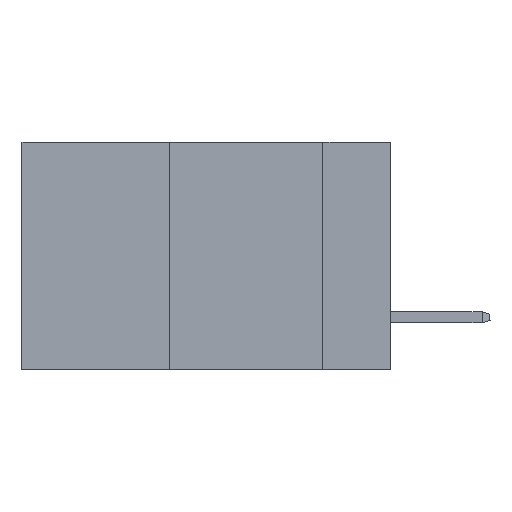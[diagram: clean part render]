
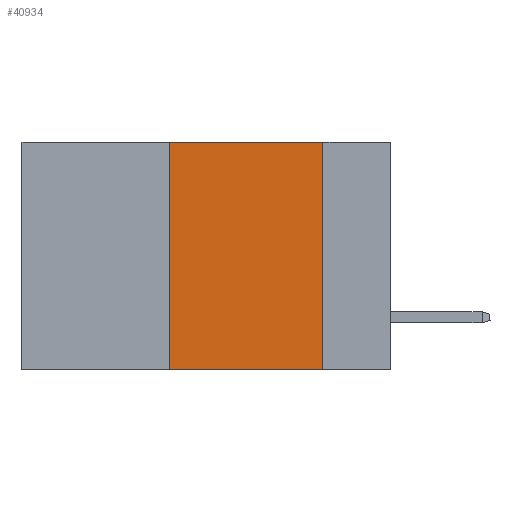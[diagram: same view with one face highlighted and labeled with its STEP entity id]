
A CAD part, left-side view. The second image highlights one B-rep face of the part: STEP entity #40934.
In plain terms, the highlighted planar face has unit normal (-1, 0, 0).
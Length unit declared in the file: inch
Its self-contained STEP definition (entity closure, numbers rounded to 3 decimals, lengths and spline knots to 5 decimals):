
#1738 = DIRECTION ( 'NONE',  ( 0., 0., 1. ) ) ;
#4378 = EDGE_CURVE ( 'NONE', #25977, #31112, #27702, .T. ) ;
#5043 = AXIS2_PLACEMENT_3D ( 'NONE', #37940, #41647, #41815 ) ;
#5925 = ORIENTED_EDGE ( 'NONE', *, *, #44887, .F. ) ;
#6386 = VECTOR ( 'NONE', #1738, 39.37008 ) ;
#9264 = VECTOR ( 'NONE', #41669, 39.37008 ) ;
#11361 = FACE_OUTER_BOUND ( 'NONE', #43266, .T. ) ;
#11776 = CARTESIAN_POINT ( 'NONE',  ( 0., 0.36, 0. ) ) ;
#13120 = VERTEX_POINT ( 'NONE', #40756 ) ;
#13201 = DIRECTION ( 'NONE',  ( 0., 0., -1. ) ) ;
#13769 = CARTESIAN_POINT ( 'NONE',  ( 0., 0.6, -0.37 ) ) ;
#13983 = CARTESIAN_POINT ( 'NONE',  ( 0., 0.11, -0.37 ) ) ;
#15597 = EDGE_CURVE ( 'NONE', #25977, #39584, #38592, .T. ) ;
#16536 = VECTOR ( 'NONE', #17822, 39.37008 ) ;
#17822 = DIRECTION ( 'NONE',  ( 0., -1., 0. ) ) ;
#18139 = ORIENTED_EDGE ( 'NONE', *, *, #44758, .F. ) ;
#21087 = ORIENTED_EDGE ( 'NONE', *, *, #15597, .T. ) ;
#23035 = LINE ( 'NONE', #26871, #9264 ) ;
#25406 = CARTESIAN_POINT ( 'NONE',  ( 0., 0.36, 0. ) ) ;
#25977 = VERTEX_POINT ( 'NONE', #27175 ) ;
#26871 = CARTESIAN_POINT ( 'NONE',  ( 0., 0.6, 0. ) ) ;
#27175 = CARTESIAN_POINT ( 'NONE',  ( 0., 0.36, -0.37 ) ) ;
#27702 = LINE ( 'NONE', #11776, #6386 ) ;
#27891 = CARTESIAN_POINT ( 'NONE',  ( 0., 0.11, 0. ) ) ;
#31112 = VERTEX_POINT ( 'NONE', #25406 ) ;
#34102 = LINE ( 'NONE', #27891, #41101 ) ;
#34661 = PLANE ( 'NONE',  #5043 ) ;
#37940 = CARTESIAN_POINT ( 'NONE',  ( 0., 0.6, 0. ) ) ;
#38592 = LINE ( 'NONE', #13769, #16536 ) ;
#39584 = VERTEX_POINT ( 'NONE', #13983 ) ;
#40756 = CARTESIAN_POINT ( 'NONE',  ( 0., 0.11, 0. ) ) ;
#40854 = ORIENTED_EDGE ( 'NONE', *, *, #4378, .F. ) ;
#40934 = ADVANCED_FACE ( 'NONE', ( #11361 ), #34661, .F. ) ;
#41101 = VECTOR ( 'NONE', #13201, 39.37008 ) ;
#41647 = DIRECTION ( 'NONE',  ( 1., 0., 0. ) ) ;
#41669 = DIRECTION ( 'NONE',  ( 0., -1., 0. ) ) ;
#41815 = DIRECTION ( 'NONE',  ( 0., 0., -1. ) ) ;
#43266 = EDGE_LOOP ( 'NONE', ( #5925, #18139, #40854, #21087 ) ) ;
#44758 = EDGE_CURVE ( 'NONE', #31112, #13120, #23035, .T. ) ;
#44887 = EDGE_CURVE ( 'NONE', #13120, #39584, #34102, .T. ) ;
